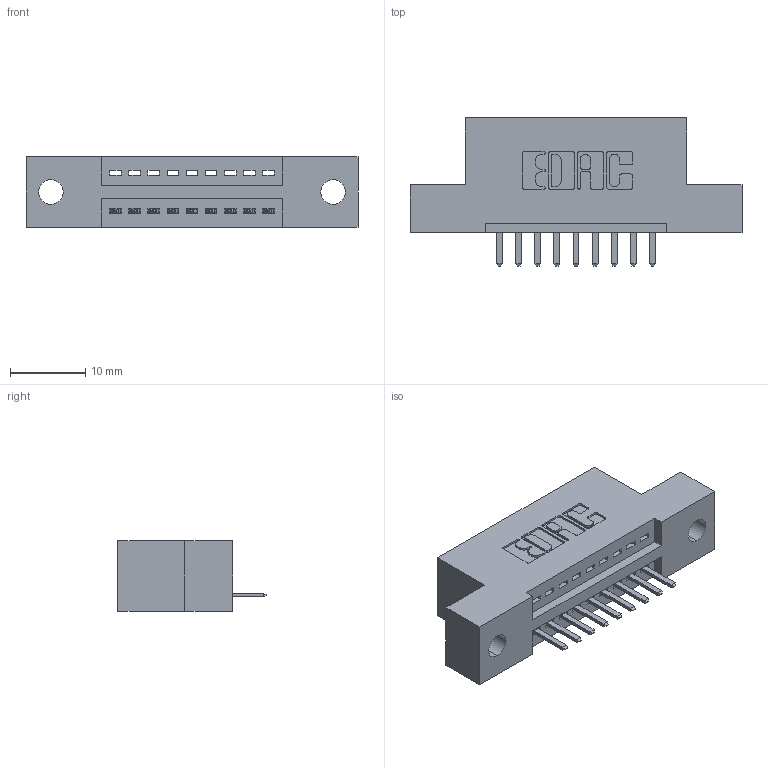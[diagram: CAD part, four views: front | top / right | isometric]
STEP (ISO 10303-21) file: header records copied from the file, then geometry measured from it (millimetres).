
FILE_DESCRIPTION (( 'STEP AP203' ), '1' );
FILE_NAME ('395-009-520-102.STEP', '2019-10-15T19:38:25', ( '' ), ( '' ), 'SwSTEP 2.0', 'SolidWorks 2016', '' );
FILE_SCHEMA (( 'CONFIG_CONTROL_DESIGN' ));
Length unit declared in the file: inch
Products named in the file (3): 345-292-001_345-293-120; 395-009-520-102; 345 Part_Flush Mounting Lugs - 0.128 Dia
Assembly tree (10 placements, depth 2):
  395-009-520-102
    345 Part_Flush Mounting Lugs - 0.128 Dia
    345-292-001_345-293-120  x9
Bounding box: 44.07 x 19.68 x 9.4 mm (x, y, z)
Volume: 3852.8 mm3; surface area: 4315.4 mm2
Topology: 10 solids, 10 shells, 684 faces, 1997 edges, 1306 vertices
Faces by surface type: plane 458, cylinder 226
Entity records: 11333 total; most frequent: CARTESIAN_POINT 1983, ORIENTED_EDGE 1914, DIRECTION 1767, EDGE_CURVE 957, LINE 785, VECTOR 785, VERTEX_POINT 634, AXIS2_PLACEMENT_3D 491
